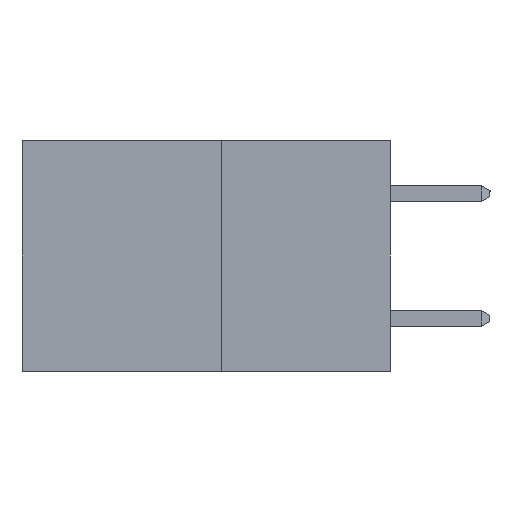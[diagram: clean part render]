
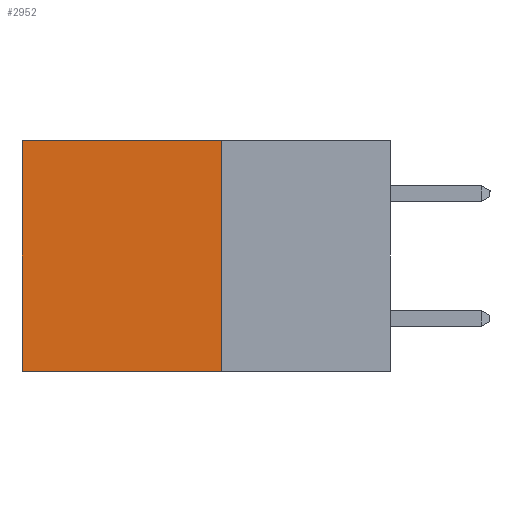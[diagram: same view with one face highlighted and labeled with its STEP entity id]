
A CAD part, left-side view. The second image highlights one B-rep face of the part: STEP entity #2952.
In plain terms, the highlighted planar face has unit normal (-1, 0, 0).
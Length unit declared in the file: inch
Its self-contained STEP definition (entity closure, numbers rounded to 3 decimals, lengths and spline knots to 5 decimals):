
#103 = CARTESIAN_POINT ( 'NONE',  ( 0.277, 0.59, -0.37 ) ) ;
#284 = VECTOR ( 'NONE', #8624, 39.37008 ) ;
#286 = DIRECTION ( 'NONE',  ( 0., 0., -1. ) ) ;
#542 = CARTESIAN_POINT ( 'NONE',  ( 0.277, 0.27, -0.37 ) ) ;
#763 = DIRECTION ( 'NONE',  ( 1., 0., 0. ) ) ;
#962 = LINE ( 'NONE', #4822, #9510 ) ;
#1108 = PLANE ( 'NONE',  #1688 ) ;
#1328 = EDGE_CURVE ( 'NONE', #5621, #4327, #2317, .T. ) ;
#1688 = AXIS2_PLACEMENT_3D ( 'NONE', #2333, #763, #286 ) ;
#1976 = CARTESIAN_POINT ( 'NONE',  ( 0.277, 0.27, 0. ) ) ;
#2005 = DIRECTION ( 'NONE',  ( 0., 0., -1. ) ) ;
#2317 = LINE ( 'NONE', #8589, #4033 ) ;
#2333 = CARTESIAN_POINT ( 'NONE',  ( 0.277, 0.27, -0.37 ) ) ;
#2459 = EDGE_CURVE ( 'NONE', #4327, #7790, #962, .T. ) ;
#2952 = ADVANCED_FACE ( 'NONE', ( #7147 ), #1108, .F. ) ;
#3251 = ORIENTED_EDGE ( 'NONE', *, *, #3740, .T. ) ;
#3684 = ORIENTED_EDGE ( 'NONE', *, *, #2459, .F. ) ;
#3740 = EDGE_CURVE ( 'NONE', #8536, #7790, #5630, .T. ) ;
#3818 = CARTESIAN_POINT ( 'NONE',  ( 0.277, 0.59, -0.37 ) ) ;
#4033 = VECTOR ( 'NONE', #2005, 39.37008 ) ;
#4037 = ORIENTED_EDGE ( 'NONE', *, *, #6138, .T. ) ;
#4327 = VERTEX_POINT ( 'NONE', #542 ) ;
#4822 = CARTESIAN_POINT ( 'NONE',  ( 0.277, 0.27, -0.37 ) ) ;
#5621 = VERTEX_POINT ( 'NONE', #10369 ) ;
#5630 = LINE ( 'NONE', #3818, #7549 ) ;
#6138 = EDGE_CURVE ( 'NONE', #5621, #8536, #9117, .T. ) ;
#6768 = ORIENTED_EDGE ( 'NONE', *, *, #1328, .F. ) ;
#7091 = DIRECTION ( 'NONE',  ( 0., 1., 0. ) ) ;
#7147 = FACE_OUTER_BOUND ( 'NONE', #7169, .T. ) ;
#7169 = EDGE_LOOP ( 'NONE', ( #3251, #3684, #6768, #4037 ) ) ;
#7549 = VECTOR ( 'NONE', #9529, 39.37008 ) ;
#7790 = VERTEX_POINT ( 'NONE', #103 ) ;
#8501 = CARTESIAN_POINT ( 'NONE',  ( 0.277, 0.59, 0. ) ) ;
#8536 = VERTEX_POINT ( 'NONE', #8501 ) ;
#8589 = CARTESIAN_POINT ( 'NONE',  ( 0.277, 0.27, -0.37 ) ) ;
#8624 = DIRECTION ( 'NONE',  ( 0., 1., 0. ) ) ;
#9117 = LINE ( 'NONE', #1976, #284 ) ;
#9510 = VECTOR ( 'NONE', #7091, 39.37008 ) ;
#9529 = DIRECTION ( 'NONE',  ( 0., 0., -1. ) ) ;
#10369 = CARTESIAN_POINT ( 'NONE',  ( 0.277, 0.27, 0. ) ) ;
